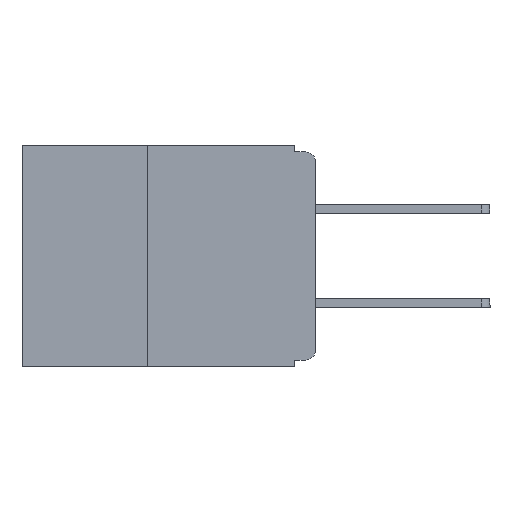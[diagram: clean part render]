
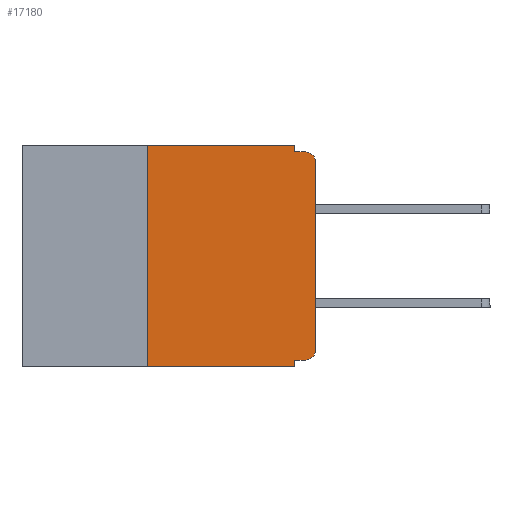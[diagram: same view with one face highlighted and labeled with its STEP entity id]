
A CAD part, left-side view. The second image highlights one B-rep face of the part: STEP entity #17180.
In plain terms, the highlighted planar face has unit normal (-1, 0, 0).
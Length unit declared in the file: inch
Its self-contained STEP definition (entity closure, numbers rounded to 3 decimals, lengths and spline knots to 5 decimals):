
#493 = CARTESIAN_POINT ( 'NONE',  ( 0., 0., -0.025 ) ) ;
#761 = VECTOR ( 'NONE', #10349, 39.37008 ) ;
#771 = CARTESIAN_POINT ( 'NONE',  ( 0., 0., -0.01 ) ) ;
#811 = CARTESIAN_POINT ( 'NONE',  ( 0., 0.015, -0.025 ) ) ;
#909 = CARTESIAN_POINT ( 'NONE',  ( 0., 0., -0.32 ) ) ;
#922 = EDGE_CURVE ( 'NONE', #5142, #9634, #17270, .T. ) ;
#1029 = VERTEX_POINT ( 'NONE', #18141 ) ;
#1385 = DIRECTION ( 'NONE',  ( 0., -1., 0. ) ) ;
#1842 = CARTESIAN_POINT ( 'NONE',  ( 0., 0.437, -0.33 ) ) ;
#2141 = CARTESIAN_POINT ( 'NONE',  ( 0., 0.031, 0. ) ) ;
#2414 = DIRECTION ( 'NONE',  ( 0., 0., -1. ) ) ;
#2432 = CARTESIAN_POINT ( 'NONE',  ( 0., 0.031, -0.33 ) ) ;
#2988 = CARTESIAN_POINT ( 'NONE',  ( 0., 0.031, -0.33 ) ) ;
#3019 = VERTEX_POINT ( 'NONE', #9469 ) ;
#3508 = LINE ( 'NONE', #909, #6763 ) ;
#3541 = CARTESIAN_POINT ( 'NONE',  ( 0., 0., -0.305 ) ) ;
#4085 = CARTESIAN_POINT ( 'NONE',  ( 0., 0.015, -0.32 ) ) ;
#4238 = DIRECTION ( 'NONE',  ( 0., 0., -1. ) ) ;
#4351 = EDGE_CURVE ( 'NONE', #12012, #12870, #16128, .T. ) ;
#4489 = VECTOR ( 'NONE', #17887, 39.37008 ) ;
#4611 = DIRECTION ( 'NONE',  ( 0., 0., -1. ) ) ;
#4709 = CIRCLE ( 'NONE', #12266, 0.015 ) ;
#4798 = LINE ( 'NONE', #1842, #17215 ) ;
#5142 = VERTEX_POINT ( 'NONE', #3541 ) ;
#5488 = ORIENTED_EDGE ( 'NONE', *, *, #12858, .F. ) ;
#5902 = EDGE_CURVE ( 'NONE', #12012, #9747, #4798, .T. ) ;
#5909 = CARTESIAN_POINT ( 'NONE',  ( 0., 0.25, -0.33 ) ) ;
#5915 = CARTESIAN_POINT ( 'NONE',  ( 0., 0., 0. ) ) ;
#6763 = VECTOR ( 'NONE', #10478, 39.37008 ) ;
#7247 = DIRECTION ( 'NONE',  ( 0., 0., 1. ) ) ;
#7496 = DIRECTION ( 'NONE',  ( 1., 0., 0. ) ) ;
#7633 = VECTOR ( 'NONE', #7247, 39.37008 ) ;
#8547 = EDGE_CURVE ( 'NONE', #19935, #16159, #12810, .T. ) ;
#8868 = DIRECTION ( 'NONE',  ( -1., 0., 0. ) ) ;
#9442 = CARTESIAN_POINT ( 'NONE',  ( 0., 0.25, 0. ) ) ;
#9469 = CARTESIAN_POINT ( 'NONE',  ( 0., 0.015, -0.01 ) ) ;
#9634 = VERTEX_POINT ( 'NONE', #493 ) ;
#9709 = EDGE_CURVE ( 'NONE', #16159, #3019, #12515, .T. ) ;
#9747 = VERTEX_POINT ( 'NONE', #2432 ) ;
#9772 = EDGE_CURVE ( 'NONE', #10369, #1029, #3508, .T. ) ;
#9777 = LINE ( 'NONE', #2988, #17785 ) ;
#10114 = LINE ( 'NONE', #20324, #13850 ) ;
#10349 = DIRECTION ( 'NONE',  ( 0., -1., 0. ) ) ;
#10369 = VERTEX_POINT ( 'NONE', #4085 ) ;
#10478 = DIRECTION ( 'NONE',  ( 0., 1., 0. ) ) ;
#11996 = DIRECTION ( 'NONE',  ( -1., 0., 0. ) ) ;
#12012 = VERTEX_POINT ( 'NONE', #19957 ) ;
#12266 = AXIS2_PLACEMENT_3D ( 'NONE', #811, #11996, #2414 ) ;
#12415 = DIRECTION ( 'NONE',  ( 0., -1., 0. ) ) ;
#12515 = LINE ( 'NONE', #771, #761 ) ;
#12603 = CIRCLE ( 'NONE', #18268, 0.015 ) ;
#12810 = LINE ( 'NONE', #13816, #17087 ) ;
#12858 = EDGE_CURVE ( 'NONE', #1029, #9747, #9777, .T. ) ;
#12870 = VERTEX_POINT ( 'NONE', #9442 ) ;
#12963 = CARTESIAN_POINT ( 'NONE',  ( 0., 0.031, -0.01 ) ) ;
#13036 = AXIS2_PLACEMENT_3D ( 'NONE', #18607, #7496, #18669 ) ;
#13816 = CARTESIAN_POINT ( 'NONE',  ( 0., 0.031, 0. ) ) ;
#13850 = VECTOR ( 'NONE', #12415, 39.37008 ) ;
#15790 = EDGE_CURVE ( 'NONE', #10369, #5142, #12603, .T. ) ;
#15919 = EDGE_CURVE ( 'NONE', #12870, #19935, #10114, .T. ) ;
#16128 = LINE ( 'NONE', #5909, #7633 ) ;
#16159 = VERTEX_POINT ( 'NONE', #12963 ) ;
#16544 = ORIENTED_EDGE ( 'NONE', *, *, #15790, .T. ) ;
#16584 = ORIENTED_EDGE ( 'NONE', *, *, #9772, .F. ) ;
#16738 = ORIENTED_EDGE ( 'NONE', *, *, #4351, .F. ) ;
#16890 = ORIENTED_EDGE ( 'NONE', *, *, #15919, .F. ) ;
#17008 = PLANE ( 'NONE',  #13036 ) ;
#17087 = VECTOR ( 'NONE', #4238, 39.37008 ) ;
#17180 = ADVANCED_FACE ( 'NONE', ( #20281 ), #17008, .F. ) ;
#17215 = VECTOR ( 'NONE', #1385, 39.37008 ) ;
#17270 = LINE ( 'NONE', #5915, #4489 ) ;
#17313 = ORIENTED_EDGE ( 'NONE', *, *, #8547, .F. ) ;
#17345 = ORIENTED_EDGE ( 'NONE', *, *, #9709, .F. ) ;
#17577 = ORIENTED_EDGE ( 'NONE', *, *, #922, .T. ) ;
#17785 = VECTOR ( 'NONE', #4611, 39.37008 ) ;
#17887 = DIRECTION ( 'NONE',  ( 0., 0., 1. ) ) ;
#18141 = CARTESIAN_POINT ( 'NONE',  ( 0., 0.031, -0.32 ) ) ;
#18268 = AXIS2_PLACEMENT_3D ( 'NONE', #18445, #8868, #19983 ) ;
#18445 = CARTESIAN_POINT ( 'NONE',  ( 0., 0.015, -0.305 ) ) ;
#18607 = CARTESIAN_POINT ( 'NONE',  ( 0., 0.437, 0. ) ) ;
#18669 = DIRECTION ( 'NONE',  ( 0., 0., -1. ) ) ;
#18972 = EDGE_LOOP ( 'NONE', ( #17577, #19541, #17345, #17313, #16890, #16738, #20264, #5488, #16584, #16544 ) ) ;
#19541 = ORIENTED_EDGE ( 'NONE', *, *, #20024, .T. ) ;
#19935 = VERTEX_POINT ( 'NONE', #2141 ) ;
#19957 = CARTESIAN_POINT ( 'NONE',  ( 0., 0.25, -0.33 ) ) ;
#19983 = DIRECTION ( 'NONE',  ( 0., 0., -1. ) ) ;
#20024 = EDGE_CURVE ( 'NONE', #9634, #3019, #4709, .T. ) ;
#20264 = ORIENTED_EDGE ( 'NONE', *, *, #5902, .T. ) ;
#20281 = FACE_OUTER_BOUND ( 'NONE', #18972, .T. ) ;
#20324 = CARTESIAN_POINT ( 'NONE',  ( 0., 0.437, 0. ) ) ;
